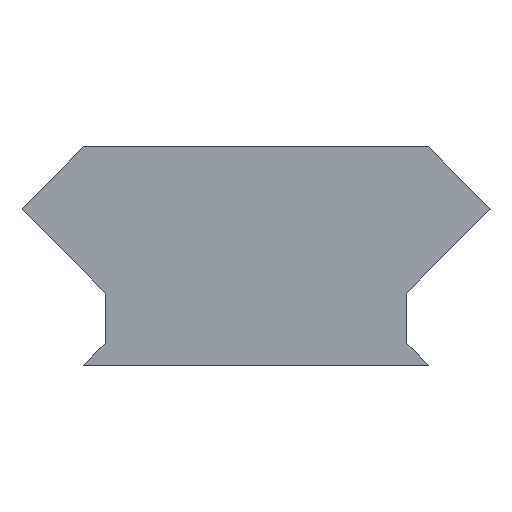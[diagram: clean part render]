
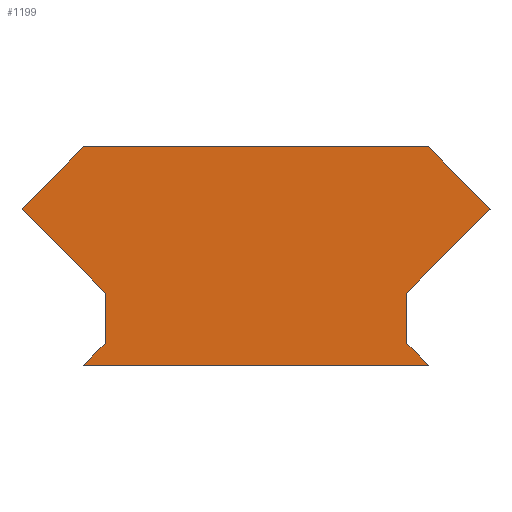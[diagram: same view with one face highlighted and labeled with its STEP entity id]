
A CAD part, left-side view. The second image highlights one B-rep face of the part: STEP entity #1199.
In plain terms, the highlighted planar face has unit normal (-1, 0, 0).
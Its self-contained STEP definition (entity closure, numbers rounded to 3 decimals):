
#15 = CARTESIAN_POINT ( 'NONE',  ( 5.5, 31.933, 20.1 ) ) ;
#56 = CARTESIAN_POINT ( 'NONE',  ( 5.5, 31.933, 30.38 ) ) ;
#60 = VECTOR ( 'NONE', #1541, 1000. ) ;
#84 = CARTESIAN_POINT ( 'NONE',  ( 5.5, 30.185, 21.848 ) ) ;
#117 = VECTOR ( 'NONE', #3058, 1000. ) ;
#126 = EDGE_CURVE ( 'NONE', #495, #826, #725, .T. ) ;
#148 = VERTEX_POINT ( 'NONE', #2977 ) ;
#164 = LINE ( 'NONE', #2035, #200 ) ;
#200 = VECTOR ( 'NONE', #639, 1000. ) ;
#202 = DIRECTION ( 'NONE',  ( 0., -0.704, 0.71 ) ) ;
#228 = DIRECTION ( 'NONE',  ( 0., 0., 1. ) ) ;
#370 = CARTESIAN_POINT ( 'NONE',  ( 5.5, 19.92, 34.633 ) ) ;
#374 = VERTEX_POINT ( 'NONE', #1249 ) ;
#393 = VECTOR ( 'NONE', #202, 1000. ) ;
#495 = VERTEX_POINT ( 'NONE', #1346 ) ;
#579 = CARTESIAN_POINT ( 'NONE',  ( 5.5, 33.724, 28.572 ) ) ;
#596 = VECTOR ( 'NONE', #1695, 1000. ) ;
#616 = ORIENTED_EDGE ( 'NONE', *, *, #2685, .F. ) ;
#639 = DIRECTION ( 'NONE',  ( 0., 0., -1. ) ) ;
#640 = EDGE_CURVE ( 'NONE', #148, #374, #809, .T. ) ;
#682 = CARTESIAN_POINT ( 'NONE',  ( 5.5, 18.59, 21.59 ) ) ;
#702 = DIRECTION ( 'NONE',  ( -1., 0., 0. ) ) ;
#725 = LINE ( 'NONE', #84, #2139 ) ;
#772 = LINE ( 'NONE', #3089, #117 ) ;
#809 = LINE ( 'NONE', #682, #393 ) ;
#826 = VERTEX_POINT ( 'NONE', #15 ) ;
#853 = CARTESIAN_POINT ( 'NONE',  ( 5.5, 30.933, 23.49 ) ) ;
#865 = ORIENTED_EDGE ( 'NONE', *, *, #2510, .T. ) ;
#946 = EDGE_CURVE ( 'NONE', #1824, #959, #1694, .T. ) ;
#959 = VERTEX_POINT ( 'NONE', #853 ) ;
#973 = CARTESIAN_POINT ( 'NONE',  ( 5.5, 35.942, 30.1 ) ) ;
#983 = CARTESIAN_POINT ( 'NONE',  ( 5.5, 15.707, 30.38 ) ) ;
#1051 = LINE ( 'NONE', #2239, #2298 ) ;
#1073 = CARTESIAN_POINT ( 'NONE',  ( 5.5, 35.053, 27.651 ) ) ;
#1199 = ADVANCED_FACE ( 'NONE', ( #2503 ), #2586, .T. ) ;
#1234 = VERTEX_POINT ( 'NONE', #983 ) ;
#1249 = CARTESIAN_POINT ( 'NONE',  ( 5.5, 12.795, 27.44 ) ) ;
#1276 = EDGE_CURVE ( 'NONE', #495, #959, #772, .T. ) ;
#1346 = CARTESIAN_POINT ( 'NONE',  ( 5.5, 30.933, 21.1 ) ) ;
#1403 = EDGE_CURVE ( 'NONE', #2470, #1705, #1051, .T. ) ;
#1523 = DIRECTION ( 'NONE',  ( 0., -0.704, -0.71 ) ) ;
#1541 = DIRECTION ( 'NONE',  ( 0., 0.704, 0.71 ) ) ;
#1542 = EDGE_CURVE ( 'NONE', #148, #1705, #164, .T. ) ;
#1587 = ORIENTED_EDGE ( 'NONE', *, *, #126, .T. ) ;
#1635 = LINE ( 'NONE', #2870, #596 ) ;
#1694 = LINE ( 'NONE', #1073, #1765 ) ;
#1695 = DIRECTION ( 'NONE',  ( 0., 1., 0. ) ) ;
#1705 = VERTEX_POINT ( 'NONE', #2812 ) ;
#1758 = ORIENTED_EDGE ( 'NONE', *, *, #1542, .F. ) ;
#1765 = VECTOR ( 'NONE', #1523, 1000. ) ;
#1767 = DIRECTION ( 'NONE',  ( 0., 0.707, -0.707 ) ) ;
#1824 = VERTEX_POINT ( 'NONE', #2157 ) ;
#1922 = LINE ( 'NONE', #2500, #2814 ) ;
#2035 = CARTESIAN_POINT ( 'NONE',  ( 5.5, 16.707, 26.513 ) ) ;
#2046 = LINE ( 'NONE', #370, #60 ) ;
#2094 = ORIENTED_EDGE ( 'NONE', *, *, #1403, .T. ) ;
#2139 = VECTOR ( 'NONE', #1767, 1000. ) ;
#2157 = CARTESIAN_POINT ( 'NONE',  ( 5.5, 34.845, 27.44 ) ) ;
#2193 = EDGE_LOOP ( 'NONE', ( #1587, #616, #2094, #1758, #2880, #2604, #2752, #865, #2475, #2859 ) ) ;
#2194 = VERTEX_POINT ( 'NONE', #56 ) ;
#2239 = CARTESIAN_POINT ( 'NONE',  ( 5.5, 23.516, 27.909 ) ) ;
#2298 = VECTOR ( 'NONE', #2679, 1000. ) ;
#2345 = VECTOR ( 'NONE', #2682, 1000. ) ;
#2470 = VERTEX_POINT ( 'NONE', #3072 ) ;
#2475 = ORIENTED_EDGE ( 'NONE', *, *, #946, .T. ) ;
#2500 = CARTESIAN_POINT ( 'NONE',  ( 5.5, 59.276, 20.1 ) ) ;
#2503 = FACE_OUTER_BOUND ( 'NONE', #2193, .T. ) ;
#2510 = EDGE_CURVE ( 'NONE', #2194, #1824, #2854, .T. ) ;
#2586 = PLANE ( 'NONE',  #2731 ) ;
#2604 = ORIENTED_EDGE ( 'NONE', *, *, #2690, .T. ) ;
#2679 = DIRECTION ( 'NONE',  ( 0., 0.707, 0.707 ) ) ;
#2682 = DIRECTION ( 'NONE',  ( 0., 0.704, -0.71 ) ) ;
#2685 = EDGE_CURVE ( 'NONE', #2470, #826, #1922, .T. ) ;
#2690 = EDGE_CURVE ( 'NONE', #374, #1234, #2046, .T. ) ;
#2731 = AXIS2_PLACEMENT_3D ( 'NONE', #973, #702, #228 ) ;
#2752 = ORIENTED_EDGE ( 'NONE', *, *, #3062, .T. ) ;
#2812 = CARTESIAN_POINT ( 'NONE',  ( 5.5, 16.707, 21.1 ) ) ;
#2814 = VECTOR ( 'NONE', #2991, 1000. ) ;
#2854 = LINE ( 'NONE', #579, #2345 ) ;
#2859 = ORIENTED_EDGE ( 'NONE', *, *, #1276, .F. ) ;
#2870 = CARTESIAN_POINT ( 'NONE',  ( 5.5, 29.881, 30.38 ) ) ;
#2880 = ORIENTED_EDGE ( 'NONE', *, *, #640, .T. ) ;
#2977 = CARTESIAN_POINT ( 'NONE',  ( 5.5, 16.707, 23.49 ) ) ;
#2991 = DIRECTION ( 'NONE',  ( 0., 1., 0. ) ) ;
#3058 = DIRECTION ( 'NONE',  ( 0., 0., 1. ) ) ;
#3062 = EDGE_CURVE ( 'NONE', #1234, #2194, #1635, .T. ) ;
#3072 = CARTESIAN_POINT ( 'NONE',  ( 5.5, 15.707, 20.1 ) ) ;
#3089 = CARTESIAN_POINT ( 'NONE',  ( 5.5, 30.933, 26.513 ) ) ;
